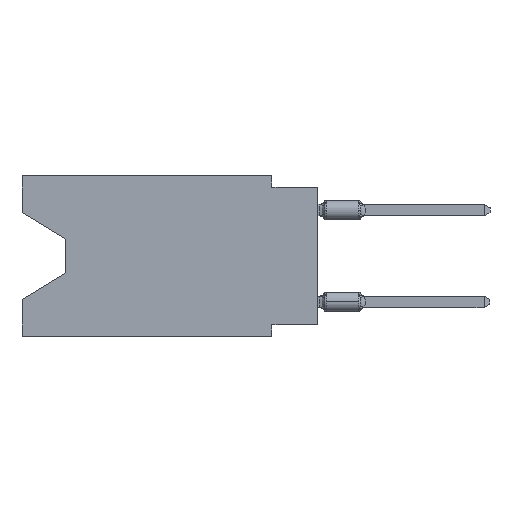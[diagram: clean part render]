
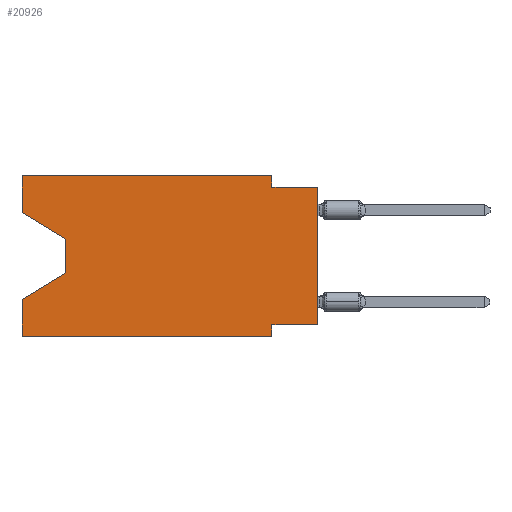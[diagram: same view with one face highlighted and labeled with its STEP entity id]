
A CAD part, left-side view. The second image highlights one B-rep face of the part: STEP entity #20926.
In plain terms, the highlighted planar face has unit normal (-1, 0, 0).
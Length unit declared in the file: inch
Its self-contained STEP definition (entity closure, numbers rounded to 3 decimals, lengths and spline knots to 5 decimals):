
#807 = VERTEX_POINT ( 'NONE', #19039 ) ;
#912 = VERTEX_POINT ( 'NONE', #10940 ) ;
#1142 = DIRECTION ( 'NONE',  ( 0., 0., -1. ) ) ;
#1538 = VERTEX_POINT ( 'NONE', #8854 ) ;
#1947 = CARTESIAN_POINT ( 'NONE',  ( 0., 0.1, -0.325 ) ) ;
#2005 = VECTOR ( 'NONE', #20551, 39.37008 ) ;
#2575 = EDGE_CURVE ( 'NONE', #11112, #8089, #7936, .T. ) ;
#4479 = EDGE_CURVE ( 'NONE', #5495, #10601, #10944, .T. ) ;
#4680 = CARTESIAN_POINT ( 'NONE',  ( 0., 0., -0.325 ) ) ;
#4894 = FACE_OUTER_BOUND ( 'NONE', #20998, .T. ) ;
#5212 = LINE ( 'NONE', #9099, #2005 ) ;
#5227 = VECTOR ( 'NONE', #17842, 39.37008 ) ;
#5343 = ORIENTED_EDGE ( 'NONE', *, *, #15714, .T. ) ;
#5495 = VERTEX_POINT ( 'NONE', #13654 ) ;
#5565 = ORIENTED_EDGE ( 'NONE', *, *, #21332, .T. ) ;
#5923 = LINE ( 'NONE', #17572, #8747 ) ;
#5992 = VECTOR ( 'NONE', #17600, 39.37008 ) ;
#6238 = CARTESIAN_POINT ( 'NONE',  ( 0., 0., -0.025 ) ) ;
#6441 = LINE ( 'NONE', #6238, #14515 ) ;
#6489 = LINE ( 'NONE', #18383, #19440 ) ;
#6504 = EDGE_CURVE ( 'NONE', #13962, #14357, #9429, .T. ) ;
#6617 = CARTESIAN_POINT ( 'NONE',  ( 0., 0.55, -0.138 ) ) ;
#6674 = ORIENTED_EDGE ( 'NONE', *, *, #15340, .F. ) ;
#6680 = VECTOR ( 'NONE', #7949, 39.37008 ) ;
#7069 = CARTESIAN_POINT ( 'NONE',  ( 0., 0.645, 0. ) ) ;
#7134 = LINE ( 'NONE', #18498, #9105 ) ;
#7621 = EDGE_CURVE ( 'NONE', #11112, #912, #8277, .T. ) ;
#7697 = CARTESIAN_POINT ( 'NONE',  ( 0., 0.645, 0. ) ) ;
#7928 = DIRECTION ( 'NONE',  ( 0., 0., 1. ) ) ;
#7936 = LINE ( 'NONE', #9877, #5227 ) ;
#7949 = DIRECTION ( 'NONE',  ( 0., 1., 0. ) ) ;
#8015 = CARTESIAN_POINT ( 'NONE',  ( 0., 0., -0.325 ) ) ;
#8089 = VERTEX_POINT ( 'NONE', #12147 ) ;
#8272 = VERTEX_POINT ( 'NONE', #8015 ) ;
#8277 = LINE ( 'NONE', #7069, #16275 ) ;
#8723 = CARTESIAN_POINT ( 'NONE',  ( 0., 0.645, 0. ) ) ;
#8747 = VECTOR ( 'NONE', #12556, 39.37008 ) ;
#8854 = CARTESIAN_POINT ( 'NONE',  ( 0., 0.1, 0. ) ) ;
#9099 = CARTESIAN_POINT ( 'NONE',  ( 0., 0.645, -0.08025 ) ) ;
#9105 = VECTOR ( 'NONE', #10181, 39.37008 ) ;
#9429 = LINE ( 'NONE', #17285, #15886 ) ;
#9454 = DIRECTION ( 'NONE',  ( 0., 0., 1. ) ) ;
#9877 = CARTESIAN_POINT ( 'NONE',  ( 0., 0.645, -0.35 ) ) ;
#10181 = DIRECTION ( 'NONE',  ( 0., 0., -1. ) ) ;
#10601 = VERTEX_POINT ( 'NONE', #8723 ) ;
#10940 = CARTESIAN_POINT ( 'NONE',  ( 0., 0.645, -0.26975 ) ) ;
#10944 = LINE ( 'NONE', #7697, #15606 ) ;
#11112 = VERTEX_POINT ( 'NONE', #16802 ) ;
#11219 = DIRECTION ( 'NONE',  ( 0., -1., 0. ) ) ;
#11583 = CARTESIAN_POINT ( 'NONE',  ( 0., 0.55, -0.212 ) ) ;
#11840 = DIRECTION ( 'NONE',  ( 0., 0., -1. ) ) ;
#12147 = CARTESIAN_POINT ( 'NONE',  ( 0., 0.1, -0.35 ) ) ;
#12391 = LINE ( 'NONE', #17855, #21289 ) ;
#12504 = ORIENTED_EDGE ( 'NONE', *, *, #16415, .F. ) ;
#12556 = DIRECTION ( 'NONE',  ( 0., -1., 0. ) ) ;
#12781 = AXIS2_PLACEMENT_3D ( 'NONE', #18416, #21558, #11840 ) ;
#13654 = CARTESIAN_POINT ( 'NONE',  ( 0., 0.645, -0.08025 ) ) ;
#13814 = ORIENTED_EDGE ( 'NONE', *, *, #7621, .F. ) ;
#13939 = ORIENTED_EDGE ( 'NONE', *, *, #16811, .F. ) ;
#13944 = ORIENTED_EDGE ( 'NONE', *, *, #4479, .F. ) ;
#13962 = VERTEX_POINT ( 'NONE', #6617 ) ;
#14357 = VERTEX_POINT ( 'NONE', #11583 ) ;
#14515 = VECTOR ( 'NONE', #11219, 39.37008 ) ;
#15248 = DIRECTION ( 'NONE',  ( 0., 0., 1. ) ) ;
#15340 = EDGE_CURVE ( 'NONE', #10601, #1538, #5923, .T. ) ;
#15342 = ORIENTED_EDGE ( 'NONE', *, *, #6504, .T. ) ;
#15551 = VERTEX_POINT ( 'NONE', #1947 ) ;
#15576 = ORIENTED_EDGE ( 'NONE', *, *, #15876, .F. ) ;
#15606 = VECTOR ( 'NONE', #7928, 39.37008 ) ;
#15714 = EDGE_CURVE ( 'NONE', #8272, #807, #12391, .T. ) ;
#15851 = LINE ( 'NONE', #17498, #5992 ) ;
#15875 = VERTEX_POINT ( 'NONE', #16439 ) ;
#15876 = EDGE_CURVE ( 'NONE', #8272, #15551, #19723, .T. ) ;
#15886 = VECTOR ( 'NONE', #1142, 39.37008 ) ;
#16275 = VECTOR ( 'NONE', #15248, 39.37008 ) ;
#16415 = EDGE_CURVE ( 'NONE', #15551, #8089, #7134, .T. ) ;
#16439 = CARTESIAN_POINT ( 'NONE',  ( 0., 0.1, -0.025 ) ) ;
#16802 = CARTESIAN_POINT ( 'NONE',  ( 0., 0.645, -0.35 ) ) ;
#16811 = EDGE_CURVE ( 'NONE', #1538, #15875, #15851, .T. ) ;
#16835 = DIRECTION ( 'NONE',  ( 0., 0.855, -0.519 ) ) ;
#17285 = CARTESIAN_POINT ( 'NONE',  ( 0., 0.55, -0.138 ) ) ;
#17498 = CARTESIAN_POINT ( 'NONE',  ( 0., 0.1, 0. ) ) ;
#17572 = CARTESIAN_POINT ( 'NONE',  ( 0., 0.645, 0. ) ) ;
#17600 = DIRECTION ( 'NONE',  ( 0., 0., -1. ) ) ;
#17723 = ORIENTED_EDGE ( 'NONE', *, *, #2575, .T. ) ;
#17842 = DIRECTION ( 'NONE',  ( 0., -1., 0. ) ) ;
#17855 = CARTESIAN_POINT ( 'NONE',  ( 0., 0., 0. ) ) ;
#18383 = CARTESIAN_POINT ( 'NONE',  ( 0., 0.55, -0.212 ) ) ;
#18416 = CARTESIAN_POINT ( 'NONE',  ( 0., 0.645, 0. ) ) ;
#18498 = CARTESIAN_POINT ( 'NONE',  ( 0., 0.1, -0.35 ) ) ;
#18503 = ORIENTED_EDGE ( 'NONE', *, *, #18598, .F. ) ;
#18513 = PLANE ( 'NONE',  #12781 ) ;
#18598 = EDGE_CURVE ( 'NONE', #15875, #807, #6441, .T. ) ;
#19039 = CARTESIAN_POINT ( 'NONE',  ( 0., 0., -0.025 ) ) ;
#19440 = VECTOR ( 'NONE', #16835, 39.37008 ) ;
#19723 = LINE ( 'NONE', #4680, #6680 ) ;
#20551 = DIRECTION ( 'NONE',  ( 0., -0.855, -0.519 ) ) ;
#20881 = ORIENTED_EDGE ( 'NONE', *, *, #21040, .T. ) ;
#20926 = ADVANCED_FACE ( 'NONE', ( #4894 ), #18513, .F. ) ;
#20998 = EDGE_LOOP ( 'NONE', ( #20881, #15342, #5565, #13814, #17723, #12504, #15576, #5343, #18503, #13939, #6674, #13944 ) ) ;
#21040 = EDGE_CURVE ( 'NONE', #5495, #13962, #5212, .T. ) ;
#21289 = VECTOR ( 'NONE', #9454, 39.37008 ) ;
#21332 = EDGE_CURVE ( 'NONE', #14357, #912, #6489, .T. ) ;
#21558 = DIRECTION ( 'NONE',  ( 1., 0., 0. ) ) ;
